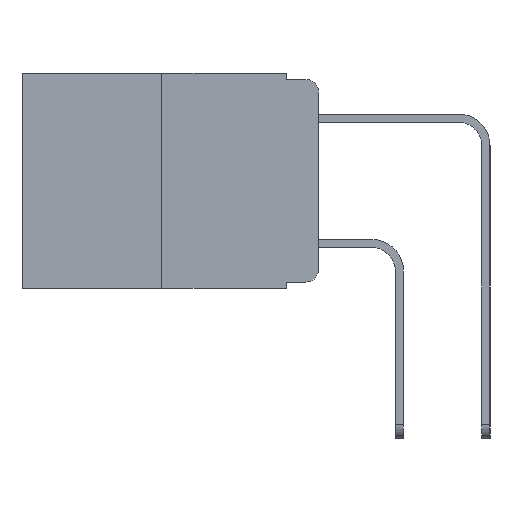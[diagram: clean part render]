
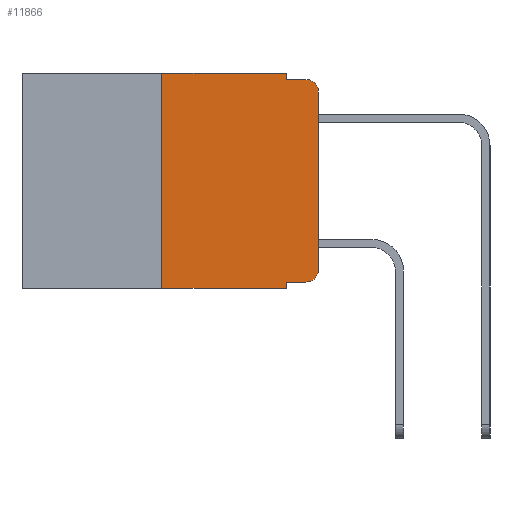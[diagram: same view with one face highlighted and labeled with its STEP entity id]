
A CAD part, left-side view. The second image highlights one B-rep face of the part: STEP entity #11866.
In plain terms, the highlighted planar face has unit normal (-1, 0, 0).
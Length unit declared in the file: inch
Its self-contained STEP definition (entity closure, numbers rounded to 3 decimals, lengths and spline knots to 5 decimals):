
#187 = VERTEX_POINT ( 'NONE', #9454 ) ;
#437 = EDGE_LOOP ( 'NONE', ( #7829, #4336, #3797, #12738, #2741, #2847, #2407, #1159, #1082, #2487 ) ) ;
#612 = EDGE_CURVE ( 'NONE', #4206, #1054, #12099, .T. ) ;
#720 = DIRECTION ( 'NONE',  ( 0., 0., 1. ) ) ;
#851 = LINE ( 'NONE', #2385, #7048 ) ;
#1046 = VECTOR ( 'NONE', #12683, 39.37008 ) ;
#1054 = VERTEX_POINT ( 'NONE', #10574 ) ;
#1082 = ORIENTED_EDGE ( 'NONE', *, *, #14201, .T. ) ;
#1159 = ORIENTED_EDGE ( 'NONE', *, *, #612, .F. ) ;
#1435 = LINE ( 'NONE', #11617, #1046 ) ;
#1437 = EDGE_CURVE ( 'NONE', #1951, #2073, #11265, .T. ) ;
#1485 = DIRECTION ( 'NONE',  ( 0., -1., 0. ) ) ;
#1522 = VERTEX_POINT ( 'NONE', #5657 ) ;
#1922 = VERTEX_POINT ( 'NONE', #10880 ) ;
#1951 = VERTEX_POINT ( 'NONE', #13014 ) ;
#2073 = VERTEX_POINT ( 'NONE', #13278 ) ;
#2232 = EDGE_CURVE ( 'NONE', #14057, #187, #1435, .T. ) ;
#2351 = CARTESIAN_POINT ( 'NONE',  ( 0., 0., -0.03 ) ) ;
#2385 = CARTESIAN_POINT ( 'NONE',  ( 0., 0.473, -0.343 ) ) ;
#2407 = ORIENTED_EDGE ( 'NONE', *, *, #5881, .T. ) ;
#2487 = ORIENTED_EDGE ( 'NONE', *, *, #13559, .T. ) ;
#2491 = VECTOR ( 'NONE', #1485, 39.37008 ) ;
#2733 = VERTEX_POINT ( 'NONE', #6437 ) ;
#2741 = ORIENTED_EDGE ( 'NONE', *, *, #3786, .F. ) ;
#2847 = ORIENTED_EDGE ( 'NONE', *, *, #1437, .F. ) ;
#3084 = EDGE_CURVE ( 'NONE', #187, #1522, #4602, .T. ) ;
#3159 = CARTESIAN_POINT ( 'NONE',  ( 0., 0.473, 0. ) ) ;
#3430 = VECTOR ( 'NONE', #9511, 39.37008 ) ;
#3445 = VECTOR ( 'NONE', #4769, 39.37008 ) ;
#3706 = DIRECTION ( 'NONE',  ( 0., -1., 0. ) ) ;
#3786 = EDGE_CURVE ( 'NONE', #2073, #14057, #11324, .T. ) ;
#3797 = ORIENTED_EDGE ( 'NONE', *, *, #3084, .F. ) ;
#3809 = CARTESIAN_POINT ( 'NONE',  ( 0., 0.051, -0.333 ) ) ;
#3894 = EDGE_CURVE ( 'NONE', #6993, #1522, #9362, .T. ) ;
#3906 = DIRECTION ( 'NONE',  ( -1., 0., 0. ) ) ;
#4206 = VERTEX_POINT ( 'NONE', #3809 ) ;
#4336 = ORIENTED_EDGE ( 'NONE', *, *, #3894, .T. ) ;
#4351 = DIRECTION ( 'NONE',  ( 0., 0., -1. ) ) ;
#4602 = LINE ( 'NONE', #7092, #10047 ) ;
#4665 = EDGE_CURVE ( 'NONE', #2733, #6993, #12112, .T. ) ;
#4769 = DIRECTION ( 'NONE',  ( 0., 0., 1. ) ) ;
#4815 = DIRECTION ( 'NONE',  ( 0., -1., 0. ) ) ;
#4855 = DIRECTION ( 'NONE',  ( 0., -1., 0. ) ) ;
#5284 = DIRECTION ( 'NONE',  ( -1., 0., 0. ) ) ;
#5567 = LINE ( 'NONE', #10265, #13742 ) ;
#5657 = CARTESIAN_POINT ( 'NONE',  ( 0., 0.02, -0.01 ) ) ;
#5881 = EDGE_CURVE ( 'NONE', #1951, #1054, #851, .T. ) ;
#6074 = AXIS2_PLACEMENT_3D ( 'NONE', #11711, #5284, #12749 ) ;
#6437 = CARTESIAN_POINT ( 'NONE',  ( 0., 0., -0.313 ) ) ;
#6993 = VERTEX_POINT ( 'NONE', #2351 ) ;
#7048 = VECTOR ( 'NONE', #4815, 39.37008 ) ;
#7092 = CARTESIAN_POINT ( 'NONE',  ( 0., 0.051, -0.01 ) ) ;
#7674 = CARTESIAN_POINT ( 'NONE',  ( 0., 0.25, 0. ) ) ;
#7829 = ORIENTED_EDGE ( 'NONE', *, *, #4665, .T. ) ;
#8010 = CARTESIAN_POINT ( 'NONE',  ( 0., 0., 0. ) ) ;
#8214 = CARTESIAN_POINT ( 'NONE',  ( 0., 0.051, 0. ) ) ;
#8452 = VECTOR ( 'NONE', #720, 39.37008 ) ;
#8966 = CARTESIAN_POINT ( 'NONE',  ( 0., 0.051, 0. ) ) ;
#9362 = CIRCLE ( 'NONE', #6074, 0.02 ) ;
#9454 = CARTESIAN_POINT ( 'NONE',  ( 0., 0.051, -0.01 ) ) ;
#9511 = DIRECTION ( 'NONE',  ( 0., 0., -1. ) ) ;
#9806 = PLANE ( 'NONE',  #13632 ) ;
#9838 = CIRCLE ( 'NONE', #12048, 0.02 ) ;
#10047 = VECTOR ( 'NONE', #3706, 39.37008 ) ;
#10265 = CARTESIAN_POINT ( 'NONE',  ( 0., 0.051, -0.333 ) ) ;
#10474 = CARTESIAN_POINT ( 'NONE',  ( 0., 0.02, -0.313 ) ) ;
#10574 = CARTESIAN_POINT ( 'NONE',  ( 0., 0.051, -0.343 ) ) ;
#10866 = DIRECTION ( 'NONE',  ( 1., 0., 0. ) ) ;
#10880 = CARTESIAN_POINT ( 'NONE',  ( 0., 0.02, -0.333 ) ) ;
#11020 = FACE_OUTER_BOUND ( 'NONE', #437, .T. ) ;
#11265 = LINE ( 'NONE', #7674, #8452 ) ;
#11324 = LINE ( 'NONE', #13594, #2491 ) ;
#11502 = DIRECTION ( 'NONE',  ( 0., 0., -1. ) ) ;
#11617 = CARTESIAN_POINT ( 'NONE',  ( 0., 0.051, 0. ) ) ;
#11711 = CARTESIAN_POINT ( 'NONE',  ( 0., 0.02, -0.03 ) ) ;
#11866 = ADVANCED_FACE ( 'NONE', ( #11020 ), #9806, .F. ) ;
#12048 = AXIS2_PLACEMENT_3D ( 'NONE', #10474, #3906, #11502 ) ;
#12099 = LINE ( 'NONE', #8214, #3430 ) ;
#12112 = LINE ( 'NONE', #8010, #3445 ) ;
#12683 = DIRECTION ( 'NONE',  ( 0., 0., -1. ) ) ;
#12738 = ORIENTED_EDGE ( 'NONE', *, *, #2232, .F. ) ;
#12749 = DIRECTION ( 'NONE',  ( 0., 0., -1. ) ) ;
#13014 = CARTESIAN_POINT ( 'NONE',  ( 0., 0.25, -0.343 ) ) ;
#13278 = CARTESIAN_POINT ( 'NONE',  ( 0., 0.25, 0. ) ) ;
#13559 = EDGE_CURVE ( 'NONE', #1922, #2733, #9838, .T. ) ;
#13594 = CARTESIAN_POINT ( 'NONE',  ( 0., 0.473, 0. ) ) ;
#13632 = AXIS2_PLACEMENT_3D ( 'NONE', #3159, #10866, #4351 ) ;
#13742 = VECTOR ( 'NONE', #4855, 39.37008 ) ;
#14057 = VERTEX_POINT ( 'NONE', #8966 ) ;
#14201 = EDGE_CURVE ( 'NONE', #4206, #1922, #5567, .T. ) ;
